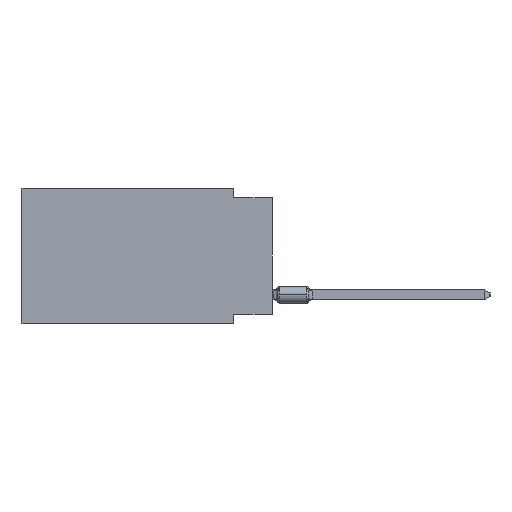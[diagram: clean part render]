
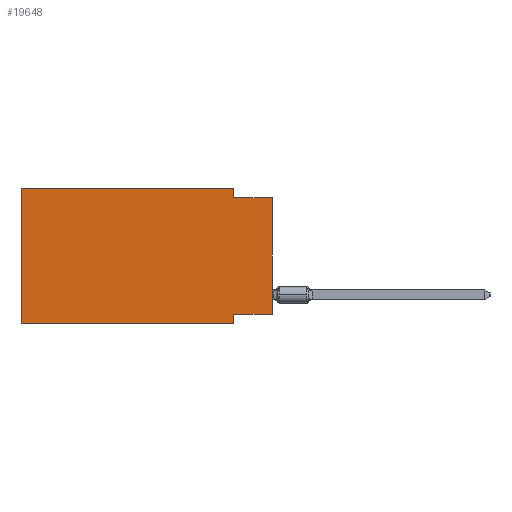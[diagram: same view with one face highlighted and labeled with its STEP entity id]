
A CAD part, left-side view. The second image highlights one B-rep face of the part: STEP entity #19648.
In plain terms, the highlighted planar face has unit normal (-1, 0, 0).
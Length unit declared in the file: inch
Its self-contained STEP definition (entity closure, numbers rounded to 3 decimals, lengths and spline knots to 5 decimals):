
#3 = VECTOR ( 'NONE', #13522, 39.37008 ) ;
#128 = CARTESIAN_POINT ( 'NONE',  ( 0., 0., -0.025 ) ) ;
#532 = VECTOR ( 'NONE', #19602, 39.37008 ) ;
#1673 = LINE ( 'NONE', #18160, #29126 ) ;
#2892 = VERTEX_POINT ( 'NONE', #11156 ) ;
#3055 = PLANE ( 'NONE',  #29400 ) ;
#3141 = CARTESIAN_POINT ( 'NONE',  ( 0., 0., 0. ) ) ;
#4142 = ORIENTED_EDGE ( 'NONE', *, *, #6416, .F. ) ;
#4387 = LINE ( 'NONE', #18425, #13869 ) ;
#4886 = EDGE_LOOP ( 'NONE', ( #9306, #23057, #8374, #11692, #18741, #7028, #4142, #27101 ) ) ;
#5587 = EDGE_CURVE ( 'NONE', #11896, #2892, #4387, .T. ) ;
#5823 = VERTEX_POINT ( 'NONE', #10239 ) ;
#5953 = VERTEX_POINT ( 'NONE', #6665 ) ;
#6416 = EDGE_CURVE ( 'NONE', #19413, #2892, #9730, .T. ) ;
#6665 = CARTESIAN_POINT ( 'NONE',  ( 0., 0.1, -0.025 ) ) ;
#6849 = DIRECTION ( 'NONE',  ( 0., -1., 0. ) ) ;
#6897 = CARTESIAN_POINT ( 'NONE',  ( 0., 0.1, 0. ) ) ;
#7028 = ORIENTED_EDGE ( 'NONE', *, *, #5587, .T. ) ;
#7659 = VERTEX_POINT ( 'NONE', #6897 ) ;
#7992 = VERTEX_POINT ( 'NONE', #8729 ) ;
#8152 = CARTESIAN_POINT ( 'NONE',  ( 0., 0.645, -0.35 ) ) ;
#8374 = ORIENTED_EDGE ( 'NONE', *, *, #26085, .F. ) ;
#8729 = CARTESIAN_POINT ( 'NONE',  ( 0., 0., -0.325 ) ) ;
#9306 = ORIENTED_EDGE ( 'NONE', *, *, #27805, .T. ) ;
#9521 = DIRECTION ( 'NONE',  ( 0., -1., 0. ) ) ;
#9730 = LINE ( 'NONE', #9880, #21305 ) ;
#9880 = CARTESIAN_POINT ( 'NONE',  ( 0., 0.1, -0.35 ) ) ;
#10195 = CARTESIAN_POINT ( 'NONE',  ( 0., 0., -0.325 ) ) ;
#10239 = CARTESIAN_POINT ( 'NONE',  ( 0., 0., -0.025 ) ) ;
#10267 = CARTESIAN_POINT ( 'NONE',  ( 0., 0.1, -0.325 ) ) ;
#10357 = EDGE_CURVE ( 'NONE', #11896, #19053, #25285, .T. ) ;
#10609 = CARTESIAN_POINT ( 'NONE',  ( 0., 0.645, 0. ) ) ;
#10812 = EDGE_CURVE ( 'NONE', #19053, #7659, #1673, .T. ) ;
#11156 = CARTESIAN_POINT ( 'NONE',  ( 0., 0.1, -0.35 ) ) ;
#11626 = VECTOR ( 'NONE', #9521, 39.37008 ) ;
#11692 = ORIENTED_EDGE ( 'NONE', *, *, #10812, .F. ) ;
#11896 = VERTEX_POINT ( 'NONE', #8152 ) ;
#12799 = EDGE_CURVE ( 'NONE', #7992, #19413, #27311, .T. ) ;
#13345 = VECTOR ( 'NONE', #25128, 39.37008 ) ;
#13522 = DIRECTION ( 'NONE',  ( 0., 0., -1. ) ) ;
#13666 = CARTESIAN_POINT ( 'NONE',  ( 0., 0.1, 0. ) ) ;
#13869 = VECTOR ( 'NONE', #6849, 39.37008 ) ;
#14553 = LINE ( 'NONE', #3141, #20210 ) ;
#14771 = FACE_OUTER_BOUND ( 'NONE', #4886, .T. ) ;
#15081 = DIRECTION ( 'NONE',  ( 1., 0., 0. ) ) ;
#16127 = LINE ( 'NONE', #13666, #3 ) ;
#16165 = EDGE_CURVE ( 'NONE', #5953, #5823, #21237, .T. ) ;
#16975 = DIRECTION ( 'NONE',  ( 0., 0., -1. ) ) ;
#16976 = CARTESIAN_POINT ( 'NONE',  ( 0., 0.645, 0. ) ) ;
#18160 = CARTESIAN_POINT ( 'NONE',  ( 0., 0.645, 0. ) ) ;
#18425 = CARTESIAN_POINT ( 'NONE',  ( 0., 0.645, -0.35 ) ) ;
#18741 = ORIENTED_EDGE ( 'NONE', *, *, #10357, .F. ) ;
#19026 = DIRECTION ( 'NONE',  ( 0., 0., 1. ) ) ;
#19053 = VERTEX_POINT ( 'NONE', #16976 ) ;
#19413 = VERTEX_POINT ( 'NONE', #10267 ) ;
#19602 = DIRECTION ( 'NONE',  ( 0., 1., 0. ) ) ;
#19648 = ADVANCED_FACE ( 'NONE', ( #14771 ), #3055, .F. ) ;
#20210 = VECTOR ( 'NONE', #19026, 39.37008 ) ;
#20643 = CARTESIAN_POINT ( 'NONE',  ( 0., 0.645, 0. ) ) ;
#21237 = LINE ( 'NONE', #128, #11626 ) ;
#21305 = VECTOR ( 'NONE', #16975, 39.37008 ) ;
#23057 = ORIENTED_EDGE ( 'NONE', *, *, #16165, .F. ) ;
#25128 = DIRECTION ( 'NONE',  ( 0., 0., 1. ) ) ;
#25285 = LINE ( 'NONE', #20643, #13345 ) ;
#26085 = EDGE_CURVE ( 'NONE', #7659, #5953, #16127, .T. ) ;
#27101 = ORIENTED_EDGE ( 'NONE', *, *, #12799, .F. ) ;
#27311 = LINE ( 'NONE', #10195, #532 ) ;
#27805 = EDGE_CURVE ( 'NONE', #7992, #5823, #14553, .T. ) ;
#28807 = DIRECTION ( 'NONE',  ( 0., 0., -1. ) ) ;
#29126 = VECTOR ( 'NONE', #30023, 39.37008 ) ;
#29400 = AXIS2_PLACEMENT_3D ( 'NONE', #10609, #15081, #28807 ) ;
#30023 = DIRECTION ( 'NONE',  ( 0., -1., 0. ) ) ;
